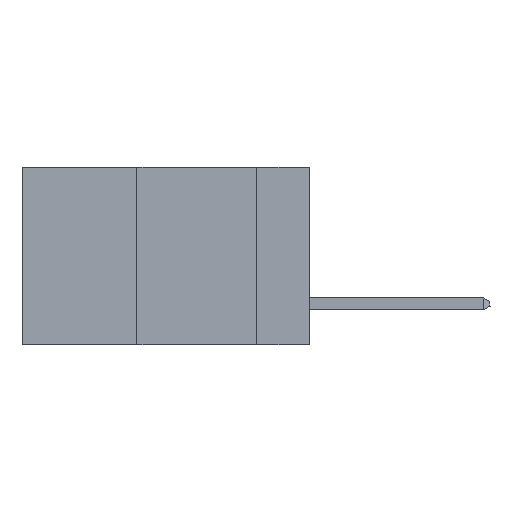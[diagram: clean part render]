
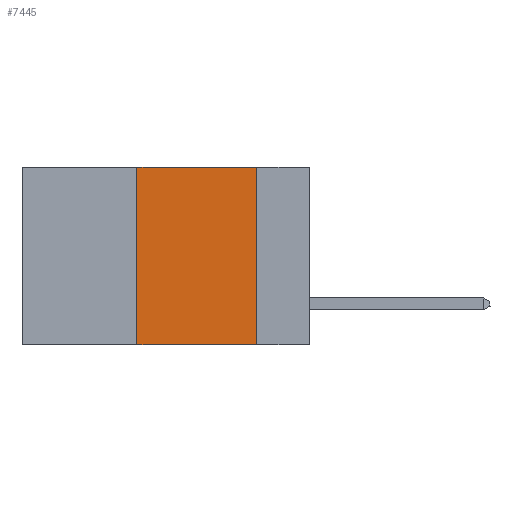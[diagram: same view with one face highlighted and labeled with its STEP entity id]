
A CAD part, left-side view. The second image highlights one B-rep face of the part: STEP entity #7445.
In plain terms, the highlighted planar face has unit normal (-1, 0, 0).
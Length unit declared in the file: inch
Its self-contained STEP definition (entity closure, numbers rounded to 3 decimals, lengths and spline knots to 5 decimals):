
#131 = VERTEX_POINT ( 'NONE', #20763 ) ;
#376 = VECTOR ( 'NONE', #8943, 39.37008 ) ;
#696 = FACE_OUTER_BOUND ( 'NONE', #2777, .T. ) ;
#1121 = DIRECTION ( 'NONE',  ( 0., -1., 0. ) ) ;
#1189 = CARTESIAN_POINT ( 'NONE',  ( 0., 0.11, -0.37 ) ) ;
#1191 = LINE ( 'NONE', #17594, #376 ) ;
#1399 = LINE ( 'NONE', #15576, #14702 ) ;
#1492 = DIRECTION ( 'NONE',  ( 0., 0., 1. ) ) ;
#2536 = ORIENTED_EDGE ( 'NONE', *, *, #13144, .F. ) ;
#2777 = EDGE_LOOP ( 'NONE', ( #16876, #2536, #5346, #17474 ) ) ;
#2932 = CARTESIAN_POINT ( 'NONE',  ( 0., 0.36, 0. ) ) ;
#4902 = DIRECTION ( 'NONE',  ( 1., 0., 0. ) ) ;
#5241 = VECTOR ( 'NONE', #1121, 39.37008 ) ;
#5346 = ORIENTED_EDGE ( 'NONE', *, *, #13634, .F. ) ;
#5911 = PLANE ( 'NONE',  #7737 ) ;
#6935 = DIRECTION ( 'NONE',  ( 0., 0., -1. ) ) ;
#7445 = ADVANCED_FACE ( 'NONE', ( #696 ), #5911, .F. ) ;
#7737 = AXIS2_PLACEMENT_3D ( 'NONE', #14346, #4902, #13404 ) ;
#8724 = EDGE_CURVE ( 'NONE', #21831, #15079, #10149, .T. ) ;
#8943 = DIRECTION ( 'NONE',  ( 0., -1., 0. ) ) ;
#10149 = LINE ( 'NONE', #18184, #5241 ) ;
#11761 = LINE ( 'NONE', #2932, #18814 ) ;
#12849 = CARTESIAN_POINT ( 'NONE',  ( 0., 0.36, -0.37 ) ) ;
#13144 = EDGE_CURVE ( 'NONE', #20901, #131, #1191, .T. ) ;
#13404 = DIRECTION ( 'NONE',  ( 0., 0., -1. ) ) ;
#13634 = EDGE_CURVE ( 'NONE', #21831, #20901, #11761, .T. ) ;
#14346 = CARTESIAN_POINT ( 'NONE',  ( 0., 0.6, 0. ) ) ;
#14702 = VECTOR ( 'NONE', #6935, 39.37008 ) ;
#15079 = VERTEX_POINT ( 'NONE', #1189 ) ;
#15576 = CARTESIAN_POINT ( 'NONE',  ( 0., 0.11, 0. ) ) ;
#16876 = ORIENTED_EDGE ( 'NONE', *, *, #16975, .F. ) ;
#16975 = EDGE_CURVE ( 'NONE', #131, #15079, #1399, .T. ) ;
#17474 = ORIENTED_EDGE ( 'NONE', *, *, #8724, .T. ) ;
#17594 = CARTESIAN_POINT ( 'NONE',  ( 0., 0.6, 0. ) ) ;
#18184 = CARTESIAN_POINT ( 'NONE',  ( 0., 0.6, -0.37 ) ) ;
#18814 = VECTOR ( 'NONE', #1492, 39.37008 ) ;
#19729 = CARTESIAN_POINT ( 'NONE',  ( 0., 0.36, 0. ) ) ;
#20763 = CARTESIAN_POINT ( 'NONE',  ( 0., 0.11, 0. ) ) ;
#20901 = VERTEX_POINT ( 'NONE', #19729 ) ;
#21831 = VERTEX_POINT ( 'NONE', #12849 ) ;
